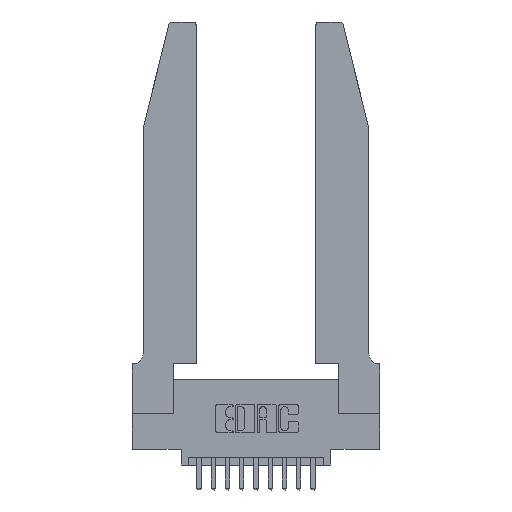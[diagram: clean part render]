
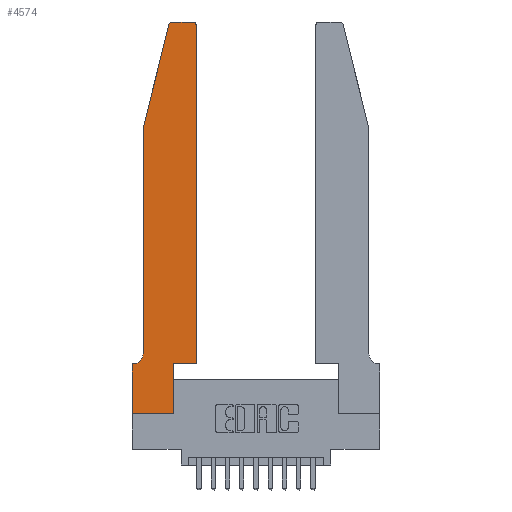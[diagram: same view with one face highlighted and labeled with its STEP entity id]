
A CAD part, top view. The second image highlights one B-rep face of the part: STEP entity #4574.
In plain terms, the highlighted planar face has unit normal (0, 0, 1).
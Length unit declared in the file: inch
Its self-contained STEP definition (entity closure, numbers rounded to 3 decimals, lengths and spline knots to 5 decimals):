
#533 = CARTESIAN_POINT ( 'NONE',  ( 0., 0.35, 0.37 ) ) ;
#562 = PLANE ( 'NONE',  #8977 ) ;
#642 = LINE ( 'NONE', #15420, #13862 ) ;
#690 = EDGE_CURVE ( 'NONE', #7336, #2629, #8177, .T. ) ;
#851 = LINE ( 'NONE', #14291, #11155 ) ;
#972 = CARTESIAN_POINT ( 'NONE',  ( 0.0755, 0.42, 0.37 ) ) ;
#1307 = VECTOR ( 'NONE', #10913, 39.37008 ) ;
#1546 = DIRECTION ( 'NONE',  ( -1., 0., 0. ) ) ;
#1909 = CARTESIAN_POINT ( 'NONE',  ( 0.25487, 2.72718, 0.37 ) ) ;
#1912 = CARTESIAN_POINT ( 'NONE',  ( 0., 0., 0.37 ) ) ;
#2511 = VERTEX_POINT ( 'NONE', #533 ) ;
#2629 = VERTEX_POINT ( 'NONE', #14477 ) ;
#2645 = VERTEX_POINT ( 'NONE', #5630 ) ;
#3038 = VECTOR ( 'NONE', #1546, 39.37008 ) ;
#3181 = DIRECTION ( 'NONE',  ( 0., 0., 1. ) ) ;
#3410 = DIRECTION ( 'NONE',  ( -1., 0., 0. ) ) ;
#3582 = CIRCLE ( 'NONE', #10127, 0.03 ) ;
#3765 = EDGE_CURVE ( 'NONE', #4999, #2511, #6475, .T. ) ;
#3905 = DIRECTION ( 'NONE',  ( 0., 0., 1. ) ) ;
#4053 = ORIENTED_EDGE ( 'NONE', *, *, #12234, .T. ) ;
#4098 = LINE ( 'NONE', #11057, #10097 ) ;
#4209 = ORIENTED_EDGE ( 'NONE', *, *, #10660, .T. ) ;
#4574 = ADVANCED_FACE ( 'NONE', ( #12471 ), #562, .T. ) ;
#4972 = CARTESIAN_POINT ( 'NONE',  ( 0.0055, 0.42, 0.37 ) ) ;
#4999 = VERTEX_POINT ( 'NONE', #15682 ) ;
#5084 = ORIENTED_EDGE ( 'NONE', *, *, #7857, .T. ) ;
#5505 = VERTEX_POINT ( 'NONE', #7524 ) ;
#5630 = CARTESIAN_POINT ( 'NONE',  ( 0.2865, 0.35, 0.37 ) ) ;
#6241 = DIRECTION ( 'NONE',  ( -1., 0., 0. ) ) ;
#6378 = ORIENTED_EDGE ( 'NONE', *, *, #3765, .T. ) ;
#6389 = EDGE_CURVE ( 'NONE', #8974, #10080, #642, .T. ) ;
#6475 = LINE ( 'NONE', #15512, #3038 ) ;
#6634 = DIRECTION ( 'NONE',  ( 0., 0., 1. ) ) ;
#6711 = DIRECTION ( 'NONE',  ( 1., 0., 0. ) ) ;
#6828 = VERTEX_POINT ( 'NONE', #972 ) ;
#6910 = CARTESIAN_POINT ( 'NONE',  ( 0., 0., 0.37 ) ) ;
#7197 = VECTOR ( 'NONE', #3410, 39.37008 ) ;
#7233 = CARTESIAN_POINT ( 'NONE',  ( 0., 0., 0.37 ) ) ;
#7235 = ORIENTED_EDGE ( 'NONE', *, *, #6389, .T. ) ;
#7297 = ORIENTED_EDGE ( 'NONE', *, *, #15489, .T. ) ;
#7336 = VERTEX_POINT ( 'NONE', #8646 ) ;
#7510 = ORIENTED_EDGE ( 'NONE', *, *, #13045, .T. ) ;
#7524 = CARTESIAN_POINT ( 'NONE',  ( 0.2865, 0., 0.37 ) ) ;
#7704 = DIRECTION ( 'NONE',  ( 0., -1., 0. ) ) ;
#7857 = EDGE_CURVE ( 'NONE', #5505, #2645, #4098, .T. ) ;
#8177 = LINE ( 'NONE', #11326, #1307 ) ;
#8304 = DIRECTION ( 'NONE',  ( 0., -1., 0. ) ) ;
#8646 = CARTESIAN_POINT ( 'NONE',  ( 0.4505, 0.35, 0.37 ) ) ;
#8949 = CARTESIAN_POINT ( 'NONE',  ( 0.0755, 2., 0.37 ) ) ;
#8974 = VERTEX_POINT ( 'NONE', #1909 ) ;
#8977 = AXIS2_PLACEMENT_3D ( 'NONE', #10896, #3181, #12163 ) ;
#9288 = ORIENTED_EDGE ( 'NONE', *, *, #13758, .T. ) ;
#9798 = EDGE_CURVE ( 'NONE', #13791, #8974, #3582, .T. ) ;
#10051 = VERTEX_POINT ( 'NONE', #6910 ) ;
#10080 = VERTEX_POINT ( 'NONE', #10846 ) ;
#10097 = VECTOR ( 'NONE', #13560, 39.37008 ) ;
#10127 = AXIS2_PLACEMENT_3D ( 'NONE', #11583, #3905, #12835 ) ;
#10216 = ORIENTED_EDGE ( 'NONE', *, *, #15917, .T. ) ;
#10253 = VECTOR ( 'NONE', #7704, 39.37008 ) ;
#10370 = LINE ( 'NONE', #7233, #13309 ) ;
#10636 = LINE ( 'NONE', #12377, #7197 ) ;
#10660 = EDGE_CURVE ( 'NONE', #2511, #10051, #11993, .T. ) ;
#10814 = ORIENTED_EDGE ( 'NONE', *, *, #9798, .T. ) ;
#10846 = CARTESIAN_POINT ( 'NONE',  ( 0.0755, 2., 0.37 ) ) ;
#10896 = CARTESIAN_POINT ( 'NONE',  ( 0., 0.35, 0.37 ) ) ;
#10913 = DIRECTION ( 'NONE',  ( 0., 1., 0. ) ) ;
#10924 = AXIS2_PLACEMENT_3D ( 'NONE', #14220, #6634, #15453 ) ;
#11057 = CARTESIAN_POINT ( 'NONE',  ( 0.2865, 0.35, 0.37 ) ) ;
#11155 = VECTOR ( 'NONE', #6711, 39.37008 ) ;
#11326 = CARTESIAN_POINT ( 'NONE',  ( 0.4505, 0.35, 0.37 ) ) ;
#11411 = CARTESIAN_POINT ( 'NONE',  ( 0.284, 2.75, 0.37 ) ) ;
#11451 = LINE ( 'NONE', #8949, #10253 ) ;
#11583 = CARTESIAN_POINT ( 'NONE',  ( 0.284, 2.72, 0.37 ) ) ;
#11605 = VECTOR ( 'NONE', #8304, 39.37008 ) ;
#11714 = DIRECTION ( 'NONE',  ( -0.239, -0.971, 0. ) ) ;
#11839 = VERTEX_POINT ( 'NONE', #15857 ) ;
#11993 = LINE ( 'NONE', #1912, #11605 ) ;
#12163 = DIRECTION ( 'NONE',  ( 1., 0., 0. ) ) ;
#12234 = EDGE_CURVE ( 'NONE', #2645, #7336, #851, .T. ) ;
#12377 = CARTESIAN_POINT ( 'NONE',  ( 0.2605, 2.75, 0.37 ) ) ;
#12409 = CIRCLE ( 'NONE', #10924, 0.03 ) ;
#12471 = FACE_OUTER_BOUND ( 'NONE', #15348, .T. ) ;
#12835 = DIRECTION ( 'NONE',  ( 1., 0., 0. ) ) ;
#13045 = EDGE_CURVE ( 'NONE', #10051, #5505, #10370, .T. ) ;
#13309 = VECTOR ( 'NONE', #14801, 39.37008 ) ;
#13493 = ORIENTED_EDGE ( 'NONE', *, *, #15584, .T. ) ;
#13560 = DIRECTION ( 'NONE',  ( 0., 1., 0. ) ) ;
#13758 = EDGE_CURVE ( 'NONE', #6828, #4999, #14584, .T. ) ;
#13791 = VERTEX_POINT ( 'NONE', #11411 ) ;
#13846 = DIRECTION ( 'NONE',  ( 0., 0., -1. ) ) ;
#13862 = VECTOR ( 'NONE', #11714, 39.37008 ) ;
#14102 = ORIENTED_EDGE ( 'NONE', *, *, #690, .T. ) ;
#14220 = CARTESIAN_POINT ( 'NONE',  ( 0.4205, 2.72, 0.37 ) ) ;
#14291 = CARTESIAN_POINT ( 'NONE',  ( 0.4505, 0.35, 0.37 ) ) ;
#14477 = CARTESIAN_POINT ( 'NONE',  ( 0.4505, 2.72, 0.37 ) ) ;
#14584 = CIRCLE ( 'NONE', #16084, 0.07 ) ;
#14801 = DIRECTION ( 'NONE',  ( 1., 0., 0. ) ) ;
#15348 = EDGE_LOOP ( 'NONE', ( #10216, #10814, #7235, #7297, #9288, #6378, #4209, #7510, #5084, #4053, #14102, #13493 ) ) ;
#15420 = CARTESIAN_POINT ( 'NONE',  ( 0.0755, 2., 0.37 ) ) ;
#15453 = DIRECTION ( 'NONE',  ( 1., 0., 0. ) ) ;
#15489 = EDGE_CURVE ( 'NONE', #10080, #6828, #11451, .T. ) ;
#15512 = CARTESIAN_POINT ( 'NONE',  ( 0.0755, 0.35, 0.37 ) ) ;
#15584 = EDGE_CURVE ( 'NONE', #2629, #11839, #12409, .T. ) ;
#15682 = CARTESIAN_POINT ( 'NONE',  ( 0.0055, 0.35, 0.37 ) ) ;
#15857 = CARTESIAN_POINT ( 'NONE',  ( 0.4205, 2.75, 0.37 ) ) ;
#15917 = EDGE_CURVE ( 'NONE', #11839, #13791, #10636, .T. ) ;
#16084 = AXIS2_PLACEMENT_3D ( 'NONE', #4972, #13846, #6241 ) ;
